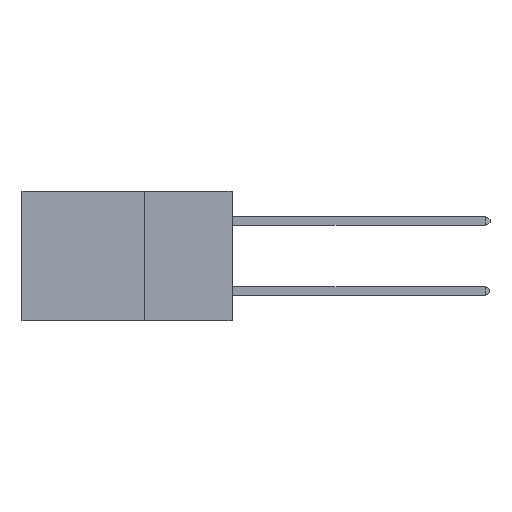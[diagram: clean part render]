
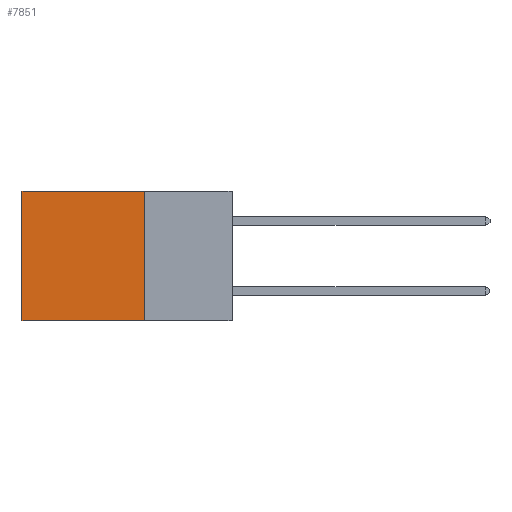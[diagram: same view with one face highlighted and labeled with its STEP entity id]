
A CAD part, left-side view. The second image highlights one B-rep face of the part: STEP entity #7851.
In plain terms, the highlighted planar face has unit normal (-1, 0, 0).
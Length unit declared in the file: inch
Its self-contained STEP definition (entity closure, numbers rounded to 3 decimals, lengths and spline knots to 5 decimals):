
#237 = ORIENTED_EDGE ( 'NONE', *, *, #14799, .F. ) ;
#581 = EDGE_CURVE ( 'NONE', #6382, #3360, #10755, .T. ) ;
#1616 = LINE ( 'NONE', #6768, #13746 ) ;
#2239 = EDGE_CURVE ( 'NONE', #2266, #3360, #8309, .T. ) ;
#2266 = VERTEX_POINT ( 'NONE', #6826 ) ;
#3360 = VERTEX_POINT ( 'NONE', #15010 ) ;
#4441 = CARTESIAN_POINT ( 'NONE',  ( 0.2875, 0.25, 0. ) ) ;
#4452 = DIRECTION ( 'NONE',  ( 0., 1., 0. ) ) ;
#4488 = CARTESIAN_POINT ( 'NONE',  ( 0.2875, 0.25, 0. ) ) ;
#4999 = CARTESIAN_POINT ( 'NONE',  ( 0.2875, 0.25, -0.37 ) ) ;
#5349 = CARTESIAN_POINT ( 'NONE',  ( 0.2875, 0.25, 0. ) ) ;
#5514 = EDGE_LOOP ( 'NONE', ( #15110, #12047, #237, #8549 ) ) ;
#5683 = PLANE ( 'NONE',  #9755 ) ;
#6382 = VERTEX_POINT ( 'NONE', #14420 ) ;
#6768 = CARTESIAN_POINT ( 'NONE',  ( 0.2875, 0.25, 0. ) ) ;
#6826 = CARTESIAN_POINT ( 'NONE',  ( 0.2875, 0.25, -0.37 ) ) ;
#7035 = CARTESIAN_POINT ( 'NONE',  ( 0.2875, 0.6, 0. ) ) ;
#7103 = VERTEX_POINT ( 'NONE', #5349 ) ;
#7851 = ADVANCED_FACE ( 'NONE', ( #14171 ), #5683, .F. ) ;
#7976 = VECTOR ( 'NONE', #13987, 39.37008 ) ;
#8047 = DIRECTION ( 'NONE',  ( 0., 0., -1. ) ) ;
#8309 = LINE ( 'NONE', #4999, #11088 ) ;
#8549 = ORIENTED_EDGE ( 'NONE', *, *, #11430, .T. ) ;
#8651 = DIRECTION ( 'NONE',  ( 0., 1., 0. ) ) ;
#9755 = AXIS2_PLACEMENT_3D ( 'NONE', #4488, #14909, #8047 ) ;
#10755 = LINE ( 'NONE', #7035, #7976 ) ;
#11088 = VECTOR ( 'NONE', #8651, 39.37008 ) ;
#11430 = EDGE_CURVE ( 'NONE', #7103, #6382, #1616, .T. ) ;
#12033 = VECTOR ( 'NONE', #12682, 39.37008 ) ;
#12047 = ORIENTED_EDGE ( 'NONE', *, *, #2239, .F. ) ;
#12682 = DIRECTION ( 'NONE',  ( 0., 0., -1. ) ) ;
#13746 = VECTOR ( 'NONE', #4452, 39.37008 ) ;
#13987 = DIRECTION ( 'NONE',  ( 0., 0., -1. ) ) ;
#14171 = FACE_OUTER_BOUND ( 'NONE', #5514, .T. ) ;
#14420 = CARTESIAN_POINT ( 'NONE',  ( 0.2875, 0.6, 0. ) ) ;
#14799 = EDGE_CURVE ( 'NONE', #7103, #2266, #15015, .T. ) ;
#14909 = DIRECTION ( 'NONE',  ( 1., 0., 0. ) ) ;
#15010 = CARTESIAN_POINT ( 'NONE',  ( 0.2875, 0.6, -0.37 ) ) ;
#15015 = LINE ( 'NONE', #4441, #12033 ) ;
#15110 = ORIENTED_EDGE ( 'NONE', *, *, #581, .T. ) ;
